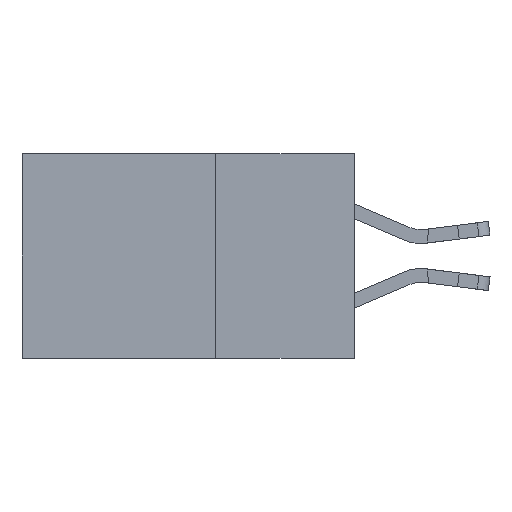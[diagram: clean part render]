
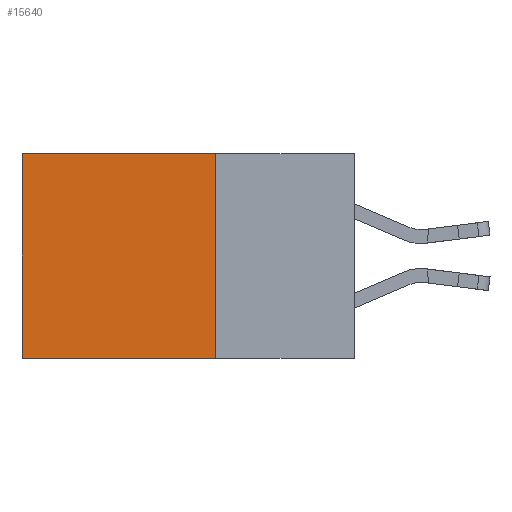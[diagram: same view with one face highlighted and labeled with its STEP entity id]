
A CAD part, left-side view. The second image highlights one B-rep face of the part: STEP entity #15640.
In plain terms, the highlighted planar face has unit normal (-1, 0, 0).
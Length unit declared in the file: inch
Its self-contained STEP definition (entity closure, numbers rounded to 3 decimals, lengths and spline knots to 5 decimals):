
#534 = ORIENTED_EDGE ( 'NONE', *, *, #18910, .T. ) ;
#1748 = EDGE_CURVE ( 'NONE', #10968, #23688, #21672, .T. ) ;
#2050 = VECTOR ( 'NONE', #22755, 39.37008 ) ;
#3525 = CARTESIAN_POINT ( 'NONE',  ( 0.298, 0.25, -0.37 ) ) ;
#3605 = AXIS2_PLACEMENT_3D ( 'NONE', #6235, #19528, #15931 ) ;
#3803 = LINE ( 'NONE', #3525, #2050 ) ;
#5677 = ORIENTED_EDGE ( 'NONE', *, *, #1748, .T. ) ;
#5845 = PLANE ( 'NONE',  #3605 ) ;
#5881 = EDGE_LOOP ( 'NONE', ( #534, #13899, #21958, #5677 ) ) ;
#6235 = CARTESIAN_POINT ( 'NONE',  ( 0.298, 0.25, 0. ) ) ;
#6672 = CARTESIAN_POINT ( 'NONE',  ( 0.298, 0.6, -0.37 ) ) ;
#7562 = EDGE_CURVE ( 'NONE', #10968, #19070, #9581, .T. ) ;
#8686 = CARTESIAN_POINT ( 'NONE',  ( 0.298, 0.6, 0. ) ) ;
#9581 = LINE ( 'NONE', #16866, #22631 ) ;
#9642 = VECTOR ( 'NONE', #17295, 39.37008 ) ;
#10968 = VERTEX_POINT ( 'NONE', #19757 ) ;
#12814 = VERTEX_POINT ( 'NONE', #6672 ) ;
#13295 = DIRECTION ( 'NONE',  ( 0., 1., 0. ) ) ;
#13899 = ORIENTED_EDGE ( 'NONE', *, *, #15825, .F. ) ;
#15640 = ADVANCED_FACE ( 'NONE', ( #23913 ), #5845, .F. ) ;
#15825 = EDGE_CURVE ( 'NONE', #19070, #12814, #3803, .T. ) ;
#15931 = DIRECTION ( 'NONE',  ( 0., 0., -1. ) ) ;
#16866 = CARTESIAN_POINT ( 'NONE',  ( 0.298, 0.25, 0. ) ) ;
#17295 = DIRECTION ( 'NONE',  ( 0., 0., -1. ) ) ;
#17771 = CARTESIAN_POINT ( 'NONE',  ( 0.298, 0.25, -0.37 ) ) ;
#18580 = LINE ( 'NONE', #22644, #9642 ) ;
#18910 = EDGE_CURVE ( 'NONE', #23688, #12814, #18580, .T. ) ;
#19070 = VERTEX_POINT ( 'NONE', #17771 ) ;
#19528 = DIRECTION ( 'NONE',  ( 1., 0., 0. ) ) ;
#19757 = CARTESIAN_POINT ( 'NONE',  ( 0.298, 0.25, 0. ) ) ;
#21259 = CARTESIAN_POINT ( 'NONE',  ( 0.298, 0.25, 0. ) ) ;
#21672 = LINE ( 'NONE', #21259, #22242 ) ;
#21958 = ORIENTED_EDGE ( 'NONE', *, *, #7562, .F. ) ;
#22242 = VECTOR ( 'NONE', #13295, 39.37008 ) ;
#22631 = VECTOR ( 'NONE', #23139, 39.37008 ) ;
#22644 = CARTESIAN_POINT ( 'NONE',  ( 0.298, 0.6, 0. ) ) ;
#22755 = DIRECTION ( 'NONE',  ( 0., 1., 0. ) ) ;
#23139 = DIRECTION ( 'NONE',  ( 0., 0., -1. ) ) ;
#23688 = VERTEX_POINT ( 'NONE', #8686 ) ;
#23913 = FACE_OUTER_BOUND ( 'NONE', #5881, .T. ) ;
